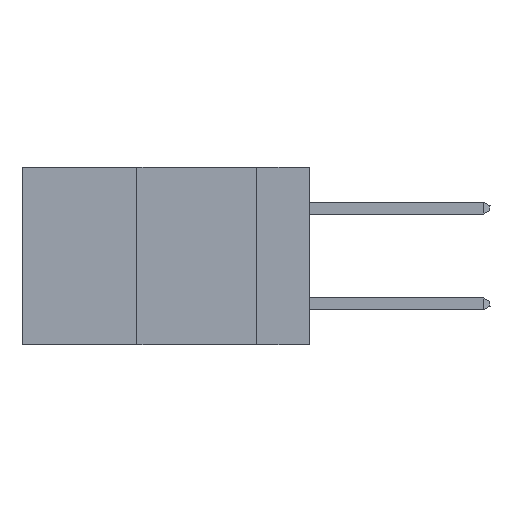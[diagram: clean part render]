
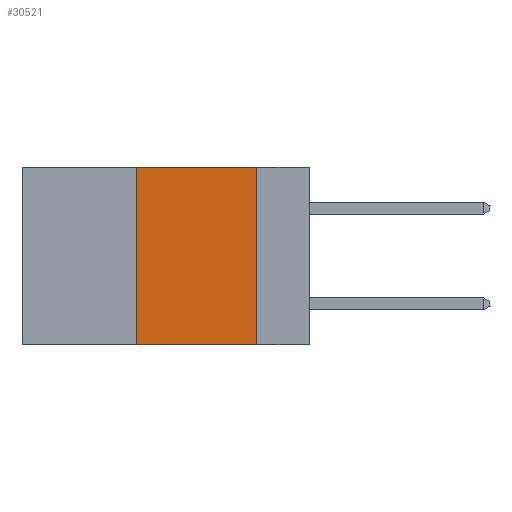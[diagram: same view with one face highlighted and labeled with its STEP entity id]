
A CAD part, left-side view. The second image highlights one B-rep face of the part: STEP entity #30521.
In plain terms, the highlighted planar face has unit normal (-1, 0, 0).
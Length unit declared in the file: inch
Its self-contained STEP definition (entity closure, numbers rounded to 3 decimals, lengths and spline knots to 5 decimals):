
#312 = DIRECTION ( 'NONE',  ( 0., 0., -1. ) ) ;
#983 = FACE_OUTER_BOUND ( 'NONE', #31076, .T. ) ;
#1527 = EDGE_CURVE ( 'NONE', #17891, #12254, #16441, .T. ) ;
#2260 = LINE ( 'NONE', #21549, #28764 ) ;
#2374 = LINE ( 'NONE', #14957, #14618 ) ;
#2480 = DIRECTION ( 'NONE',  ( 1., 0., 0. ) ) ;
#4524 = EDGE_CURVE ( 'NONE', #22197, #31984, #2260, .T. ) ;
#4620 = DIRECTION ( 'NONE',  ( 0., 0., 1. ) ) ;
#5798 = VECTOR ( 'NONE', #312, 39.37008 ) ;
#8595 = EDGE_CURVE ( 'NONE', #17891, #22197, #2374, .T. ) ;
#9559 = CARTESIAN_POINT ( 'NONE',  ( 0., 0.11, 0. ) ) ;
#10551 = AXIS2_PLACEMENT_3D ( 'NONE', #28062, #2480, #20561 ) ;
#10650 = CARTESIAN_POINT ( 'NONE',  ( 0., 0.11, 0. ) ) ;
#10672 = DIRECTION ( 'NONE',  ( 0., -1., 0. ) ) ;
#11427 = DIRECTION ( 'NONE',  ( 0., -1., 0. ) ) ;
#12254 = VERTEX_POINT ( 'NONE', #26705 ) ;
#14618 = VECTOR ( 'NONE', #4620, 39.37008 ) ;
#14957 = CARTESIAN_POINT ( 'NONE',  ( 0., 0.36, 0. ) ) ;
#16129 = ORIENTED_EDGE ( 'NONE', *, *, #27998, .F. ) ;
#16441 = LINE ( 'NONE', #25577, #29077 ) ;
#17891 = VERTEX_POINT ( 'NONE', #30258 ) ;
#18601 = ORIENTED_EDGE ( 'NONE', *, *, #4524, .F. ) ;
#20561 = DIRECTION ( 'NONE',  ( 0., 0., -1. ) ) ;
#21475 = ORIENTED_EDGE ( 'NONE', *, *, #1527, .T. ) ;
#21549 = CARTESIAN_POINT ( 'NONE',  ( 0., 0.6, 0. ) ) ;
#22197 = VERTEX_POINT ( 'NONE', #23437 ) ;
#23437 = CARTESIAN_POINT ( 'NONE',  ( 0., 0.36, 0. ) ) ;
#25551 = PLANE ( 'NONE',  #10551 ) ;
#25577 = CARTESIAN_POINT ( 'NONE',  ( 0., 0.6, -0.37 ) ) ;
#26705 = CARTESIAN_POINT ( 'NONE',  ( 0., 0.11, -0.37 ) ) ;
#27003 = LINE ( 'NONE', #10650, #5798 ) ;
#27998 = EDGE_CURVE ( 'NONE', #31984, #12254, #27003, .T. ) ;
#28062 = CARTESIAN_POINT ( 'NONE',  ( 0., 0.6, 0. ) ) ;
#28764 = VECTOR ( 'NONE', #11427, 39.37008 ) ;
#29077 = VECTOR ( 'NONE', #10672, 39.37008 ) ;
#29608 = ORIENTED_EDGE ( 'NONE', *, *, #8595, .F. ) ;
#30258 = CARTESIAN_POINT ( 'NONE',  ( 0., 0.36, -0.37 ) ) ;
#30521 = ADVANCED_FACE ( 'NONE', ( #983 ), #25551, .F. ) ;
#31076 = EDGE_LOOP ( 'NONE', ( #16129, #18601, #29608, #21475 ) ) ;
#31984 = VERTEX_POINT ( 'NONE', #9559 ) ;
